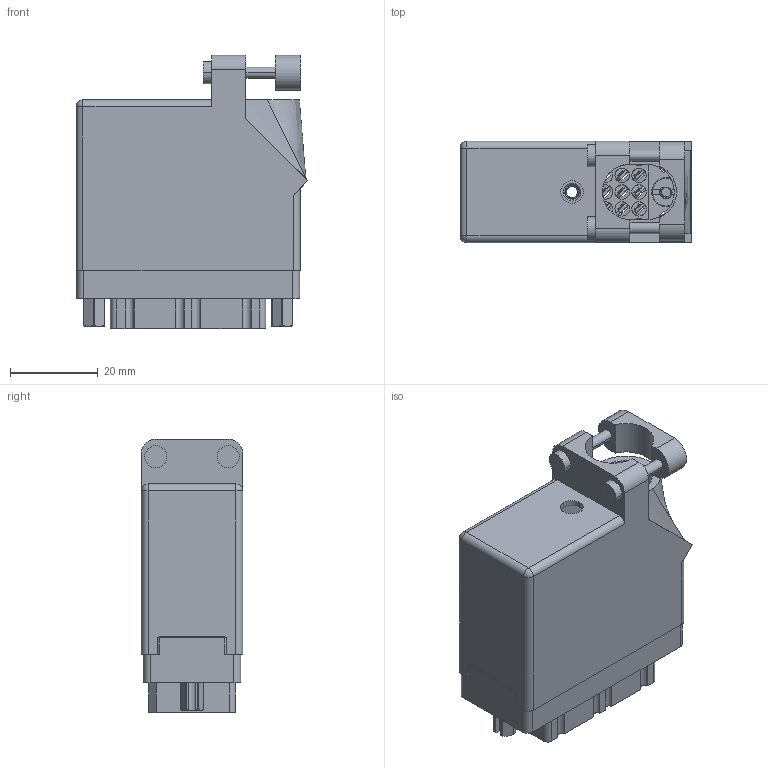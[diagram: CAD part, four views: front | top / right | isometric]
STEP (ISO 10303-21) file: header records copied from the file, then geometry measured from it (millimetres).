
FILE_DESCRIPTION (( 'STEP AP203' ), '1' );
FILE_NAME ('519-036-500-412.STEP', '2020-09-09T20:16:58', ( '' ), ( '' ), 'SwSTEP 2.0', 'SolidWorks 2020', '' );
FILE_SCHEMA (( 'CONFIG_CONTROL_DESIGN' ));
Length unit declared in the file: inch
Products named in the file (8): 516-221-038-102_038; 516-292-001_500 Contact; 516-221-038-102_039; 516-252-035-100_516-252-035-100; 519-036-500-412; 519 Receptacle Insulator_036; 516-252-021-102_038; 516-230-001_Plastic - 038 Top Entry
Assembly tree (43 placements, depth 2):
  519-036-500-412
    519 Receptacle Insulator_036
    516-292-001_500 Contact  x36
    516-252-035-100_516-252-035-100
    516-252-021-102_038  x2
    516-221-038-102_038
    516-221-038-102_039
    516-230-001_Plastic - 038 Top Entry
Bounding box: 52.85 x 23.11 x 62.26 mm (x, y, z)
Volume: 23676.5 mm3; surface area: 36001 mm2
Topology: 43 solids, 43 shells, 3874 faces, 11183 edges, 7414 vertices
Faces by surface type: plane 2254, cylinder 1321, bspline 253, cone 44, sphere 2
Entity records: 47433 total; most frequent: CARTESIAN_POINT 14234, ORIENTED_EDGE 6774, DIRECTION 6366, EDGE_CURVE 3387, VECTOR 2288, LINE 2288, VERTEX_POINT 2244, AXIS2_PLACEMENT_3D 2039
